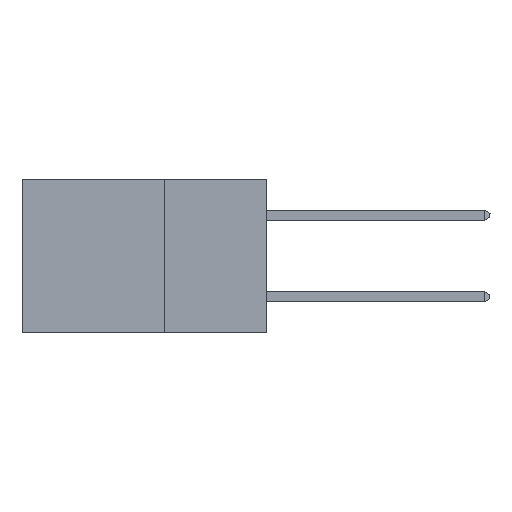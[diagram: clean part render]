
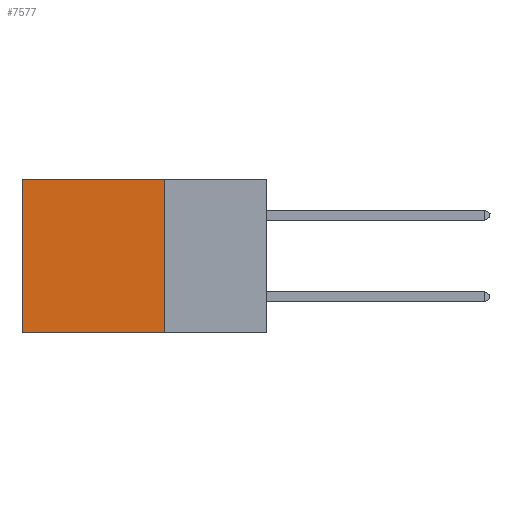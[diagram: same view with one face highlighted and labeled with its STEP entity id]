
A CAD part, left-side view. The second image highlights one B-rep face of the part: STEP entity #7577.
In plain terms, the highlighted planar face has unit normal (-1, 0, 0).
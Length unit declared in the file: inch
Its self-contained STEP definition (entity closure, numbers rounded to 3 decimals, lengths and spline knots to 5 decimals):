
#98 = DIRECTION ( 'NONE',  ( 0., 0., -1. ) ) ;
#219 = CARTESIAN_POINT ( 'NONE',  ( 0.2875, 0.25, 0. ) ) ;
#894 = LINE ( 'NONE', #1100, #4571 ) ;
#1012 = VECTOR ( 'NONE', #7258, 39.37008 ) ;
#1100 = CARTESIAN_POINT ( 'NONE',  ( 0.2875, 0.25, -0.375 ) ) ;
#1849 = LINE ( 'NONE', #10607, #1012 ) ;
#2293 = LINE ( 'NONE', #11370, #8451 ) ;
#2455 = CARTESIAN_POINT ( 'NONE',  ( 0.2875, 0.25, 0. ) ) ;
#2606 = DIRECTION ( 'NONE',  ( 1., 0., 0. ) ) ;
#4166 = ORIENTED_EDGE ( 'NONE', *, *, #6973, .T. ) ;
#4437 = EDGE_CURVE ( 'NONE', #7086, #8453, #2293, .T. ) ;
#4571 = VECTOR ( 'NONE', #13583, 39.37008 ) ;
#5191 = ORIENTED_EDGE ( 'NONE', *, *, #10455, .F. ) ;
#5732 = CARTESIAN_POINT ( 'NONE',  ( 0.2875, 0.25, -0.375 ) ) ;
#5933 = DIRECTION ( 'NONE',  ( 0., 0., -1. ) ) ;
#6025 = CARTESIAN_POINT ( 'NONE',  ( 0.2875, 0.6, -0.375 ) ) ;
#6074 = VERTEX_POINT ( 'NONE', #9041 ) ;
#6973 = EDGE_CURVE ( 'NONE', #10640, #7086, #7116, .T. ) ;
#7086 = VERTEX_POINT ( 'NONE', #8667 ) ;
#7116 = LINE ( 'NONE', #219, #9329 ) ;
#7258 = DIRECTION ( 'NONE',  ( 0., 0., -1. ) ) ;
#7577 = ADVANCED_FACE ( 'NONE', ( #12061 ), #7949, .F. ) ;
#7949 = PLANE ( 'NONE',  #12492 ) ;
#8002 = ORIENTED_EDGE ( 'NONE', *, *, #4437, .T. ) ;
#8451 = VECTOR ( 'NONE', #98, 39.37008 ) ;
#8453 = VERTEX_POINT ( 'NONE', #6025 ) ;
#8667 = CARTESIAN_POINT ( 'NONE',  ( 0.2875, 0.6, 0. ) ) ;
#9041 = CARTESIAN_POINT ( 'NONE',  ( 0.2875, 0.25, -0.375 ) ) ;
#9329 = VECTOR ( 'NONE', #12904, 39.37008 ) ;
#10455 = EDGE_CURVE ( 'NONE', #10640, #6074, #1849, .T. ) ;
#10491 = EDGE_CURVE ( 'NONE', #6074, #8453, #894, .T. ) ;
#10607 = CARTESIAN_POINT ( 'NONE',  ( 0.2875, 0.25, -0.375 ) ) ;
#10640 = VERTEX_POINT ( 'NONE', #2455 ) ;
#11160 = ORIENTED_EDGE ( 'NONE', *, *, #10491, .F. ) ;
#11370 = CARTESIAN_POINT ( 'NONE',  ( 0.2875, 0.6, -0.375 ) ) ;
#12061 = FACE_OUTER_BOUND ( 'NONE', #12086, .T. ) ;
#12086 = EDGE_LOOP ( 'NONE', ( #8002, #11160, #5191, #4166 ) ) ;
#12492 = AXIS2_PLACEMENT_3D ( 'NONE', #5732, #2606, #5933 ) ;
#12904 = DIRECTION ( 'NONE',  ( 0., 1., 0. ) ) ;
#13583 = DIRECTION ( 'NONE',  ( 0., 1., 0. ) ) ;
